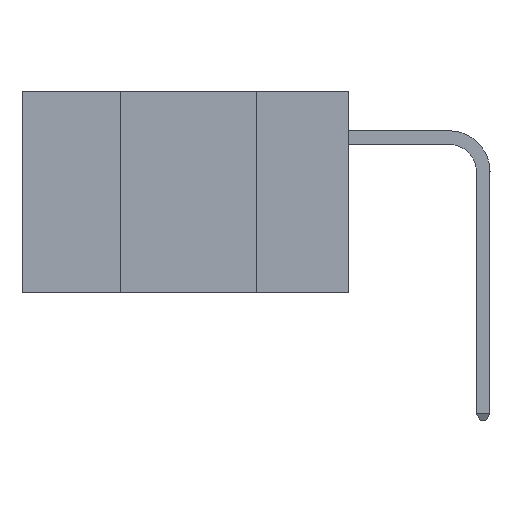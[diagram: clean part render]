
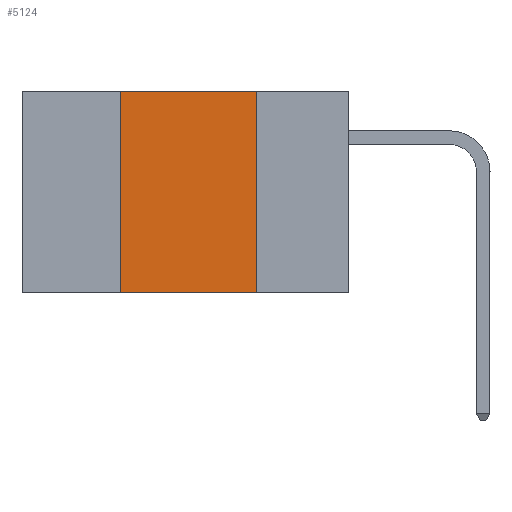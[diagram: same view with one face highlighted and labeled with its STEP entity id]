
A CAD part, left-side view. The second image highlights one B-rep face of the part: STEP entity #5124.
In plain terms, the highlighted planar face has unit normal (-1, 0, 0).
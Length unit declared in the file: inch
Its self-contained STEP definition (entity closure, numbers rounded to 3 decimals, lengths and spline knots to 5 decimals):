
#1819 = DIRECTION ( 'NONE',  ( 0., -1., 0. ) ) ;
#1904 = VERTEX_POINT ( 'NONE', #6122 ) ;
#2108 = CARTESIAN_POINT ( 'NONE',  ( 0., 0.42, -0.37 ) ) ;
#2533 = ORIENTED_EDGE ( 'NONE', *, *, #20511, .F. ) ;
#2555 = VECTOR ( 'NONE', #18291, 39.37008 ) ;
#3614 = VERTEX_POINT ( 'NONE', #8881 ) ;
#4639 = ORIENTED_EDGE ( 'NONE', *, *, #17886, .F. ) ;
#5124 = ADVANCED_FACE ( 'NONE', ( #23148 ), #19158, .F. ) ;
#6122 = CARTESIAN_POINT ( 'NONE',  ( 0., 0.42, 0. ) ) ;
#6694 = LINE ( 'NONE', #9532, #7868 ) ;
#7018 = VECTOR ( 'NONE', #1819, 39.37008 ) ;
#7034 = LINE ( 'NONE', #16400, #2555 ) ;
#7235 = EDGE_LOOP ( 'NONE', ( #4639, #15248, #2533, #22515 ) ) ;
#7785 = LINE ( 'NONE', #23735, #18369 ) ;
#7868 = VECTOR ( 'NONE', #20751, 39.37008 ) ;
#7919 = DIRECTION ( 'NONE',  ( 1., 0., 0. ) ) ;
#8539 = VERTEX_POINT ( 'NONE', #24251 ) ;
#8551 = EDGE_CURVE ( 'NONE', #1904, #3614, #21368, .T. ) ;
#8881 = CARTESIAN_POINT ( 'NONE',  ( 0., 0.17, 0. ) ) ;
#9532 = CARTESIAN_POINT ( 'NONE',  ( 0., 0.6, -0.37 ) ) ;
#10663 = DIRECTION ( 'NONE',  ( 0., 0., -1. ) ) ;
#13142 = CARTESIAN_POINT ( 'NONE',  ( 0., 0.6, 0. ) ) ;
#13505 = CARTESIAN_POINT ( 'NONE',  ( 0., 0.6, 0. ) ) ;
#15248 = ORIENTED_EDGE ( 'NONE', *, *, #8551, .F. ) ;
#15359 = AXIS2_PLACEMENT_3D ( 'NONE', #13505, #7919, #21030 ) ;
#15605 = EDGE_CURVE ( 'NONE', #20779, #8539, #6694, .T. ) ;
#16400 = CARTESIAN_POINT ( 'NONE',  ( 0., 0.42, 0. ) ) ;
#17886 = EDGE_CURVE ( 'NONE', #3614, #8539, #7785, .T. ) ;
#18291 = DIRECTION ( 'NONE',  ( 0., 0., 1. ) ) ;
#18369 = VECTOR ( 'NONE', #10663, 39.37008 ) ;
#19158 = PLANE ( 'NONE',  #15359 ) ;
#20511 = EDGE_CURVE ( 'NONE', #20779, #1904, #7034, .T. ) ;
#20751 = DIRECTION ( 'NONE',  ( 0., -1., 0. ) ) ;
#20779 = VERTEX_POINT ( 'NONE', #2108 ) ;
#21030 = DIRECTION ( 'NONE',  ( 0., 0., -1. ) ) ;
#21368 = LINE ( 'NONE', #13142, #7018 ) ;
#22515 = ORIENTED_EDGE ( 'NONE', *, *, #15605, .T. ) ;
#23148 = FACE_OUTER_BOUND ( 'NONE', #7235, .T. ) ;
#23735 = CARTESIAN_POINT ( 'NONE',  ( 0., 0.17, 0. ) ) ;
#24251 = CARTESIAN_POINT ( 'NONE',  ( 0., 0.17, -0.37 ) ) ;
